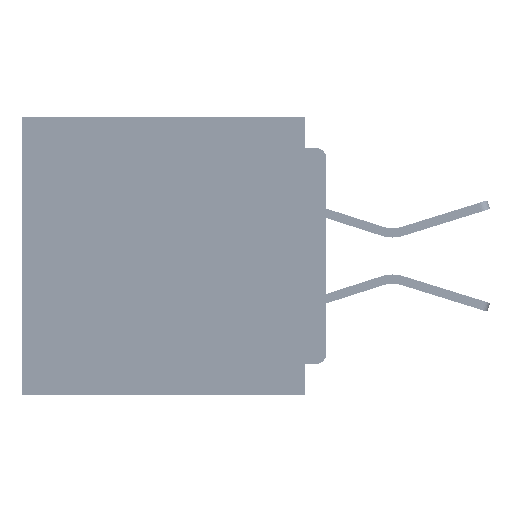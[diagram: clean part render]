
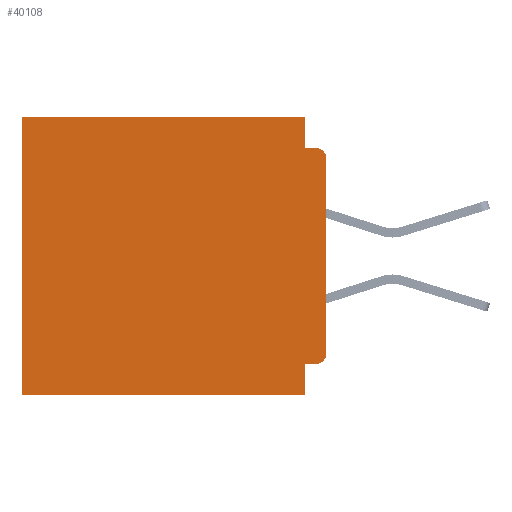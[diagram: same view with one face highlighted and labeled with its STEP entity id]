
A CAD part, left-side view. The second image highlights one B-rep face of the part: STEP entity #40108.
In plain terms, the highlighted planar face has unit normal (-1, 0, 0).
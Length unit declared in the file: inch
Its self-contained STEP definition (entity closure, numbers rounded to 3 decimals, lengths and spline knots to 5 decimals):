
#1323 = EDGE_CURVE ( 'NONE', #33563, #42960, #23996, .T. ) ;
#1357 = EDGE_CURVE ( 'NONE', #55827, #42960, #47807, .T. ) ;
#1543 = CARTESIAN_POINT ( 'NONE',  ( 0.3, 0.031, -0.4 ) ) ;
#3644 = CARTESIAN_POINT ( 'NONE',  ( 0.3, 0.031, -0.4 ) ) ;
#4770 = CARTESIAN_POINT ( 'NONE',  ( 0.3, 0., -0.34 ) ) ;
#5182 = ORIENTED_EDGE ( 'NONE', *, *, #43721, .T. ) ;
#5858 = ORIENTED_EDGE ( 'NONE', *, *, #1357, .T. ) ;
#6336 = CARTESIAN_POINT ( 'NONE',  ( 0.3, 0., 0. ) ) ;
#6400 = CARTESIAN_POINT ( 'NONE',  ( 0.3, 0.015, -0.045 ) ) ;
#7282 = VECTOR ( 'NONE', #41646, 39.37008 ) ;
#8000 = CARTESIAN_POINT ( 'NONE',  ( 0.3, 0.015, -0.355 ) ) ;
#8399 = VERTEX_POINT ( 'NONE', #46580 ) ;
#10317 = EDGE_CURVE ( 'NONE', #8399, #35729, #53588, .T. ) ;
#10640 = ORIENTED_EDGE ( 'NONE', *, *, #10317, .T. ) ;
#10691 = AXIS2_PLACEMENT_3D ( 'NONE', #42270, #11827, #47371 ) ;
#11441 = DIRECTION ( 'NONE',  ( 0., 1., 0. ) ) ;
#11579 = EDGE_CURVE ( 'NONE', #61732, #33563, #46042, .T. ) ;
#11676 = VECTOR ( 'NONE', #11441, 39.37008 ) ;
#11827 = DIRECTION ( 'NONE',  ( -1., 0., 0. ) ) ;
#12136 = VECTOR ( 'NONE', #13887, 39.37008 ) ;
#12508 = CARTESIAN_POINT ( 'NONE',  ( 0.3, 0.031, 0. ) ) ;
#13887 = DIRECTION ( 'NONE',  ( 0., 0., -1. ) ) ;
#14883 = CARTESIAN_POINT ( 'NONE',  ( 0.3, 0., -0.4 ) ) ;
#15152 = EDGE_CURVE ( 'NONE', #55827, #54507, #38497, .T. ) ;
#15319 = DIRECTION ( 'NONE',  ( 0., 0., -1. ) ) ;
#15840 = CARTESIAN_POINT ( 'NONE',  ( 0.3, 0.015, -0.06 ) ) ;
#17243 = PLANE ( 'NONE',  #21587 ) ;
#21587 = AXIS2_PLACEMENT_3D ( 'NONE', #52809, #57865, #27530 ) ;
#22474 = CARTESIAN_POINT ( 'NONE',  ( 0.3, 0.437, -0.4 ) ) ;
#22835 = DIRECTION ( 'NONE',  ( 0., 0., -1. ) ) ;
#23483 = ORIENTED_EDGE ( 'NONE', *, *, #1323, .F. ) ;
#23578 = DIRECTION ( 'NONE',  ( 0., 0., -1. ) ) ;
#23757 = VECTOR ( 'NONE', #34899, 39.37008 ) ;
#23996 = LINE ( 'NONE', #42511, #7282 ) ;
#24145 = VECTOR ( 'NONE', #35102, 39.37008 ) ;
#25432 = FACE_OUTER_BOUND ( 'NONE', #28644, .T. ) ;
#27530 = DIRECTION ( 'NONE',  ( 0., 0., -1. ) ) ;
#27922 = CARTESIAN_POINT ( 'NONE',  ( 0.3, 0.031, -0.045 ) ) ;
#28644 = EDGE_LOOP ( 'NONE', ( #65041, #5858, #23483, #44176, #35379, #10640, #33762, #59064, #31322, #5182 ) ) ;
#28861 = EDGE_CURVE ( 'NONE', #46318, #44975, #37264, .T. ) ;
#29273 = DIRECTION ( 'NONE',  ( -1., 0., 0. ) ) ;
#31322 = ORIENTED_EDGE ( 'NONE', *, *, #28861, .F. ) ;
#32550 = EDGE_CURVE ( 'NONE', #35626, #35729, #39267, .T. ) ;
#33563 = VERTEX_POINT ( 'NONE', #27922 ) ;
#33762 = ORIENTED_EDGE ( 'NONE', *, *, #32550, .F. ) ;
#34899 = DIRECTION ( 'NONE',  ( 0., 1., 0. ) ) ;
#35102 = DIRECTION ( 'NONE',  ( 0., 1., 0. ) ) ;
#35379 = ORIENTED_EDGE ( 'NONE', *, *, #44958, .T. ) ;
#35626 = VERTEX_POINT ( 'NONE', #1543 ) ;
#35729 = VERTEX_POINT ( 'NONE', #22474 ) ;
#36882 = VECTOR ( 'NONE', #15319, 39.37008 ) ;
#37264 = LINE ( 'NONE', #54868, #23757 ) ;
#37596 = LINE ( 'NONE', #3644, #12136 ) ;
#38497 = LINE ( 'NONE', #55931, #36882 ) ;
#38761 = LINE ( 'NONE', #6336, #11676 ) ;
#38916 = CARTESIAN_POINT ( 'NONE',  ( 0.3, 0.031, 0. ) ) ;
#39267 = LINE ( 'NONE', #14883, #24145 ) ;
#40095 = VECTOR ( 'NONE', #22835, 39.37008 ) ;
#40108 = ADVANCED_FACE ( 'NONE', ( #25432 ), #17243, .F. ) ;
#41646 = DIRECTION ( 'NONE',  ( 0., -1., 0. ) ) ;
#41891 = EDGE_CURVE ( 'NONE', #44975, #35626, #37596, .T. ) ;
#41898 = CARTESIAN_POINT ( 'NONE',  ( 0.3, 0.031, -0.355 ) ) ;
#42270 = CARTESIAN_POINT ( 'NONE',  ( 0.3, 0.015, -0.34 ) ) ;
#42511 = CARTESIAN_POINT ( 'NONE',  ( 0.3, 0., -0.045 ) ) ;
#42843 = VECTOR ( 'NONE', #23578, 39.37008 ) ;
#42960 = VERTEX_POINT ( 'NONE', #6400 ) ;
#43051 = CARTESIAN_POINT ( 'NONE',  ( 0.3, 0.437, -0.4 ) ) ;
#43721 = EDGE_CURVE ( 'NONE', #46318, #54507, #61100, .T. ) ;
#44176 = ORIENTED_EDGE ( 'NONE', *, *, #11579, .F. ) ;
#44958 = EDGE_CURVE ( 'NONE', #61732, #8399, #38761, .T. ) ;
#44975 = VERTEX_POINT ( 'NONE', #41898 ) ;
#46042 = LINE ( 'NONE', #38916, #42843 ) ;
#46318 = VERTEX_POINT ( 'NONE', #8000 ) ;
#46580 = CARTESIAN_POINT ( 'NONE',  ( 0.3, 0.437, 0. ) ) ;
#47371 = DIRECTION ( 'NONE',  ( 0., 0., -1. ) ) ;
#47807 = CIRCLE ( 'NONE', #58452, 0.015 ) ;
#52809 = CARTESIAN_POINT ( 'NONE',  ( 0.3, 0., -0.4 ) ) ;
#53588 = LINE ( 'NONE', #43051, #40095 ) ;
#54218 = CARTESIAN_POINT ( 'NONE',  ( 0.3, 0., -0.06 ) ) ;
#54507 = VERTEX_POINT ( 'NONE', #4770 ) ;
#54868 = CARTESIAN_POINT ( 'NONE',  ( 0.3, 0., -0.355 ) ) ;
#55827 = VERTEX_POINT ( 'NONE', #54218 ) ;
#55931 = CARTESIAN_POINT ( 'NONE',  ( 0.3, 0., -0.4 ) ) ;
#57865 = DIRECTION ( 'NONE',  ( 1., 0., 0. ) ) ;
#58452 = AXIS2_PLACEMENT_3D ( 'NONE', #15840, #29273, #59969 ) ;
#59064 = ORIENTED_EDGE ( 'NONE', *, *, #41891, .F. ) ;
#59969 = DIRECTION ( 'NONE',  ( 0., 0., -1. ) ) ;
#61100 = CIRCLE ( 'NONE', #10691, 0.015 ) ;
#61732 = VERTEX_POINT ( 'NONE', #12508 ) ;
#65041 = ORIENTED_EDGE ( 'NONE', *, *, #15152, .F. ) ;
